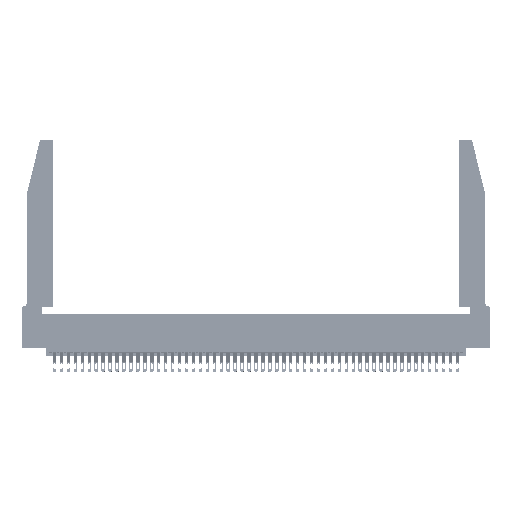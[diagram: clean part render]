
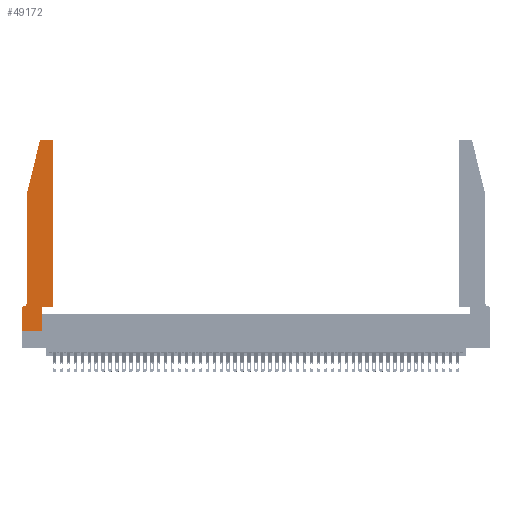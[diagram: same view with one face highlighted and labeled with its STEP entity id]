
A CAD part, top view. The second image highlights one B-rep face of the part: STEP entity #49172.
In plain terms, the highlighted planar face has unit normal (0, 0, 1).
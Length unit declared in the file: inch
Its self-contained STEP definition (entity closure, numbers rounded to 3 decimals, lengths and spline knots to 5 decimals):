
#508 = ORIENTED_EDGE ( 'NONE', *, *, #31129, .T. ) ;
#672 = DIRECTION ( 'NONE',  ( 1., 0., 0. ) ) ;
#987 = CARTESIAN_POINT ( 'NONE',  ( 0.0755, 2., 0.37 ) ) ;
#1096 = VECTOR ( 'NONE', #46146, 39.37008 ) ;
#1590 = VECTOR ( 'NONE', #33098, 39.37008 ) ;
#1647 = DIRECTION ( 'NONE',  ( 0., -1., 0. ) ) ;
#2254 = VERTEX_POINT ( 'NONE', #40786 ) ;
#2796 = CARTESIAN_POINT ( 'NONE',  ( 0.0055, 0.42, 0.37 ) ) ;
#3222 = ORIENTED_EDGE ( 'NONE', *, *, #27737, .T. ) ;
#3300 = VECTOR ( 'NONE', #14417, 39.37008 ) ;
#3698 = CARTESIAN_POINT ( 'NONE',  ( 0.0755, 2., 0.37 ) ) ;
#4817 = DIRECTION ( 'NONE',  ( 0., 1., 0. ) ) ;
#4871 = CARTESIAN_POINT ( 'NONE',  ( 0.0755, 0.42, 0.37 ) ) ;
#6072 = EDGE_CURVE ( 'NONE', #2254, #25737, #9829, .T. ) ;
#7170 = CIRCLE ( 'NONE', #9158, 0.07 ) ;
#8129 = ORIENTED_EDGE ( 'NONE', *, *, #15888, .T. ) ;
#8481 = DIRECTION ( 'NONE',  ( 0., 0., 1. ) ) ;
#9158 = AXIS2_PLACEMENT_3D ( 'NONE', #2796, #21907, #30031 ) ;
#9829 = LINE ( 'NONE', #47670, #16360 ) ;
#10030 = EDGE_CURVE ( 'NONE', #43777, #31887, #42001, .T. ) ;
#10200 = CARTESIAN_POINT ( 'NONE',  ( 0.4505, 0.35, 0.37 ) ) ;
#10434 = CARTESIAN_POINT ( 'NONE',  ( 0.0755, 0.35, 0.37 ) ) ;
#10655 = DIRECTION ( 'NONE',  ( 1., 0., 0. ) ) ;
#10942 = VECTOR ( 'NONE', #25360, 39.37008 ) ;
#11207 = EDGE_CURVE ( 'NONE', #16647, #21834, #29974, .T. ) ;
#11240 = AXIS2_PLACEMENT_3D ( 'NONE', #39397, #35085, #38736 ) ;
#12274 = DIRECTION ( 'NONE',  ( 1., 0., 0. ) ) ;
#13246 = DIRECTION ( 'NONE',  ( 0., 0., 1. ) ) ;
#13678 = LINE ( 'NONE', #22228, #14258 ) ;
#13730 = CARTESIAN_POINT ( 'NONE',  ( 0.284, 2.72, 0.37 ) ) ;
#14258 = VECTOR ( 'NONE', #48977, 39.37008 ) ;
#14417 = DIRECTION ( 'NONE',  ( -1., 0., 0. ) ) ;
#15888 = EDGE_CURVE ( 'NONE', #31887, #42628, #21890, .T. ) ;
#16360 = VECTOR ( 'NONE', #1647, 39.37008 ) ;
#16647 = VERTEX_POINT ( 'NONE', #10200 ) ;
#17110 = CARTESIAN_POINT ( 'NONE',  ( 0.25487, 2.72718, 0.37 ) ) ;
#17811 = EDGE_CURVE ( 'NONE', #25737, #21861, #47930, .T. ) ;
#17812 = CARTESIAN_POINT ( 'NONE',  ( 0.284, 2.75, 0.37 ) ) ;
#20756 = DIRECTION ( 'NONE',  ( 1., 0., 0. ) ) ;
#21174 = EDGE_CURVE ( 'NONE', #24874, #30367, #13678, .T. ) ;
#21834 = VERTEX_POINT ( 'NONE', #37571 ) ;
#21861 = VERTEX_POINT ( 'NONE', #33937 ) ;
#21890 = CIRCLE ( 'NONE', #33400, 0.03 ) ;
#21907 = DIRECTION ( 'NONE',  ( 0., 0., -1. ) ) ;
#22228 = CARTESIAN_POINT ( 'NONE',  ( 0.0755, 2., 0.37 ) ) ;
#22987 = ORIENTED_EDGE ( 'NONE', *, *, #17811, .T. ) ;
#24874 = VERTEX_POINT ( 'NONE', #3698 ) ;
#25360 = DIRECTION ( 'NONE',  ( 0., 1., 0. ) ) ;
#25524 = CARTESIAN_POINT ( 'NONE',  ( 0.4505, 0.35, 0.37 ) ) ;
#25737 = VERTEX_POINT ( 'NONE', #44657 ) ;
#25791 = CARTESIAN_POINT ( 'NONE',  ( 0.4505, 0.35, 0.37 ) ) ;
#27111 = LINE ( 'NONE', #10434, #3300 ) ;
#27112 = CARTESIAN_POINT ( 'NONE',  ( 0.2865, 0.35, 0.37 ) ) ;
#27380 = VERTEX_POINT ( 'NONE', #46507 ) ;
#27737 = EDGE_CURVE ( 'NONE', #30367, #27380, #7170, .T. ) ;
#29775 = CARTESIAN_POINT ( 'NONE',  ( 0.2605, 2.75, 0.37 ) ) ;
#29974 = LINE ( 'NONE', #25524, #10942 ) ;
#30031 = DIRECTION ( 'NONE',  ( -1., 0., 0. ) ) ;
#30367 = VERTEX_POINT ( 'NONE', #4871 ) ;
#30420 = AXIS2_PLACEMENT_3D ( 'NONE', #41830, #8481, #12274 ) ;
#30970 = VERTEX_POINT ( 'NONE', #27112 ) ;
#31129 = EDGE_CURVE ( 'NONE', #21861, #30970, #39479, .T. ) ;
#31887 = VERTEX_POINT ( 'NONE', #17812 ) ;
#32709 = EDGE_CURVE ( 'NONE', #30970, #16647, #32857, .T. ) ;
#32857 = LINE ( 'NONE', #25791, #48962 ) ;
#33098 = DIRECTION ( 'NONE',  ( -1., 0., 0. ) ) ;
#33400 = AXIS2_PLACEMENT_3D ( 'NONE', #13730, #13246, #20756 ) ;
#33937 = CARTESIAN_POINT ( 'NONE',  ( 0.2865, 0., 0.37 ) ) ;
#34215 = EDGE_CURVE ( 'NONE', #21834, #43777, #34497, .T. ) ;
#34497 = CIRCLE ( 'NONE', #11240, 0.03 ) ;
#34575 = CARTESIAN_POINT ( 'NONE',  ( 0., 0., 0.37 ) ) ;
#35023 = ORIENTED_EDGE ( 'NONE', *, *, #47164, .T. ) ;
#35085 = DIRECTION ( 'NONE',  ( 0., 0., 1. ) ) ;
#35263 = CARTESIAN_POINT ( 'NONE',  ( 0.4205, 2.75, 0.37 ) ) ;
#37060 = ORIENTED_EDGE ( 'NONE', *, *, #6072, .T. ) ;
#37571 = CARTESIAN_POINT ( 'NONE',  ( 0.4505, 2.72, 0.37 ) ) ;
#38403 = ORIENTED_EDGE ( 'NONE', *, *, #32709, .T. ) ;
#38736 = DIRECTION ( 'NONE',  ( 1., 0., 0. ) ) ;
#39397 = CARTESIAN_POINT ( 'NONE',  ( 0.4205, 2.72, 0.37 ) ) ;
#39479 = LINE ( 'NONE', #46852, #41248 ) ;
#40166 = VECTOR ( 'NONE', #672, 39.37008 ) ;
#40382 = EDGE_LOOP ( 'NONE', ( #44082, #8129, #35023, #44758, #3222, #45142, #37060, #22987, #508, #38403, #41923, #41993 ) ) ;
#40786 = CARTESIAN_POINT ( 'NONE',  ( 0., 0.35, 0.37 ) ) ;
#41248 = VECTOR ( 'NONE', #4817, 39.37008 ) ;
#41524 = LINE ( 'NONE', #987, #1096 ) ;
#41663 = PLANE ( 'NONE',  #30420 ) ;
#41830 = CARTESIAN_POINT ( 'NONE',  ( 0., 0.35, 0.37 ) ) ;
#41923 = ORIENTED_EDGE ( 'NONE', *, *, #11207, .T. ) ;
#41993 = ORIENTED_EDGE ( 'NONE', *, *, #34215, .T. ) ;
#42001 = LINE ( 'NONE', #29775, #1590 ) ;
#42056 = FACE_OUTER_BOUND ( 'NONE', #40382, .T. ) ;
#42628 = VERTEX_POINT ( 'NONE', #17110 ) ;
#42762 = EDGE_CURVE ( 'NONE', #27380, #2254, #27111, .T. ) ;
#43777 = VERTEX_POINT ( 'NONE', #35263 ) ;
#44082 = ORIENTED_EDGE ( 'NONE', *, *, #10030, .T. ) ;
#44657 = CARTESIAN_POINT ( 'NONE',  ( 0., 0., 0.37 ) ) ;
#44758 = ORIENTED_EDGE ( 'NONE', *, *, #21174, .T. ) ;
#45142 = ORIENTED_EDGE ( 'NONE', *, *, #42762, .T. ) ;
#46146 = DIRECTION ( 'NONE',  ( -0.239, -0.971, 0. ) ) ;
#46507 = CARTESIAN_POINT ( 'NONE',  ( 0.0055, 0.35, 0.37 ) ) ;
#46852 = CARTESIAN_POINT ( 'NONE',  ( 0.2865, 0.35, 0.37 ) ) ;
#47164 = EDGE_CURVE ( 'NONE', #42628, #24874, #41524, .T. ) ;
#47670 = CARTESIAN_POINT ( 'NONE',  ( 0., 0., 0.37 ) ) ;
#47930 = LINE ( 'NONE', #34575, #40166 ) ;
#48962 = VECTOR ( 'NONE', #10655, 39.37008 ) ;
#48977 = DIRECTION ( 'NONE',  ( 0., -1., 0. ) ) ;
#49172 = ADVANCED_FACE ( 'NONE', ( #42056 ), #41663, .T. ) ;
